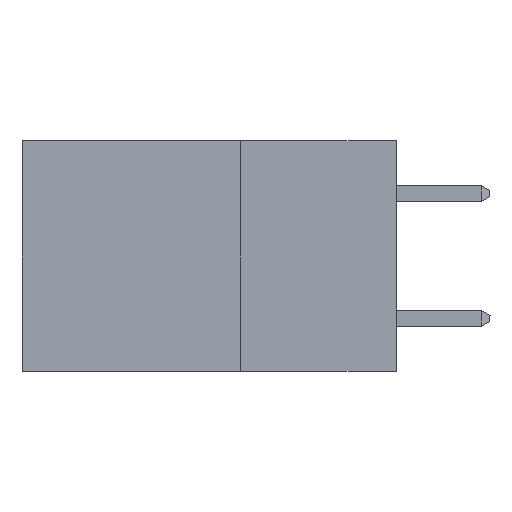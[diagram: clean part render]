
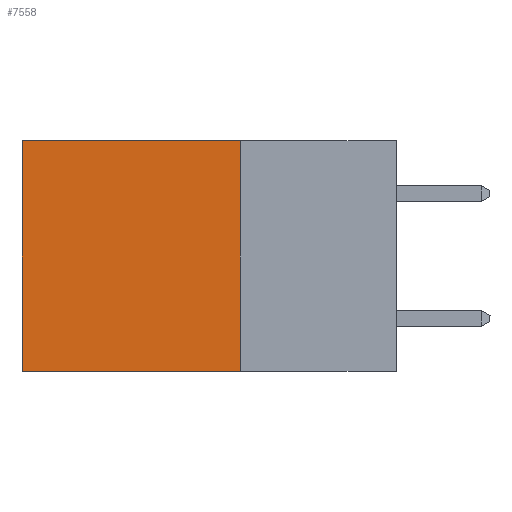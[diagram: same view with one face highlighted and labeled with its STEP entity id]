
A CAD part, left-side view. The second image highlights one B-rep face of the part: STEP entity #7558.
In plain terms, the highlighted planar face has unit normal (-1, 0, 0).
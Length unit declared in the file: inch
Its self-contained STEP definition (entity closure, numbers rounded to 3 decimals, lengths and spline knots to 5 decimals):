
#764 = LINE ( 'NONE', #8801, #4580 ) ;
#1144 = CARTESIAN_POINT ( 'NONE',  ( 0.2615, 0.25, -0.37 ) ) ;
#1654 = EDGE_CURVE ( 'NONE', #11725, #10632, #10644, .T. ) ;
#1902 = EDGE_CURVE ( 'NONE', #8868, #3682, #12857, .T. ) ;
#2535 = EDGE_CURVE ( 'NONE', #10632, #3682, #5913, .T. ) ;
#3682 = VERTEX_POINT ( 'NONE', #14457 ) ;
#3807 = FACE_OUTER_BOUND ( 'NONE', #13834, .T. ) ;
#3854 = DIRECTION ( 'NONE',  ( 0., 0., -1. ) ) ;
#4062 = DIRECTION ( 'NONE',  ( 1., 0., 0. ) ) ;
#4379 = PLANE ( 'NONE',  #11492 ) ;
#4390 = ORIENTED_EDGE ( 'NONE', *, *, #2535, .F. ) ;
#4580 = VECTOR ( 'NONE', #8824, 39.37008 ) ;
#4657 = ORIENTED_EDGE ( 'NONE', *, *, #13824, .T. ) ;
#4905 = CARTESIAN_POINT ( 'NONE',  ( 0.2615, 0.25, -0.37 ) ) ;
#5159 = VECTOR ( 'NONE', #11287, 39.37008 ) ;
#5913 = LINE ( 'NONE', #11354, #5159 ) ;
#6182 = DIRECTION ( 'NONE',  ( 0., 0., -1. ) ) ;
#6322 = VECTOR ( 'NONE', #12268, 39.37008 ) ;
#6917 = CARTESIAN_POINT ( 'NONE',  ( 0.2615, 0.25, -0.37 ) ) ;
#7323 = VECTOR ( 'NONE', #6182, 39.37008 ) ;
#7558 = ADVANCED_FACE ( 'NONE', ( #3807 ), #4379, .F. ) ;
#8801 = CARTESIAN_POINT ( 'NONE',  ( 0.2615, 0.25, 0. ) ) ;
#8824 = DIRECTION ( 'NONE',  ( 0., 1., 0. ) ) ;
#8868 = VERTEX_POINT ( 'NONE', #9393 ) ;
#9309 = ORIENTED_EDGE ( 'NONE', *, *, #1654, .F. ) ;
#9393 = CARTESIAN_POINT ( 'NONE',  ( 0.2615, 0.6, 0. ) ) ;
#10347 = ORIENTED_EDGE ( 'NONE', *, *, #1902, .T. ) ;
#10632 = VERTEX_POINT ( 'NONE', #1144 ) ;
#10644 = LINE ( 'NONE', #4905, #7323 ) ;
#11287 = DIRECTION ( 'NONE',  ( 0., 1., 0. ) ) ;
#11354 = CARTESIAN_POINT ( 'NONE',  ( 0.2615, 0.25, -0.37 ) ) ;
#11492 = AXIS2_PLACEMENT_3D ( 'NONE', #6917, #4062, #3854 ) ;
#11725 = VERTEX_POINT ( 'NONE', #15296 ) ;
#12268 = DIRECTION ( 'NONE',  ( 0., 0., -1. ) ) ;
#12674 = CARTESIAN_POINT ( 'NONE',  ( 0.2615, 0.6, -0.37 ) ) ;
#12857 = LINE ( 'NONE', #12674, #6322 ) ;
#13824 = EDGE_CURVE ( 'NONE', #11725, #8868, #764, .T. ) ;
#13834 = EDGE_LOOP ( 'NONE', ( #10347, #4390, #9309, #4657 ) ) ;
#14457 = CARTESIAN_POINT ( 'NONE',  ( 0.2615, 0.6, -0.37 ) ) ;
#15296 = CARTESIAN_POINT ( 'NONE',  ( 0.2615, 0.25, 0. ) ) ;
